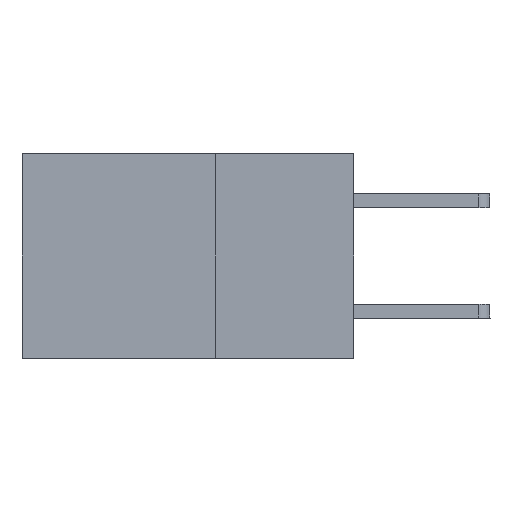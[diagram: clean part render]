
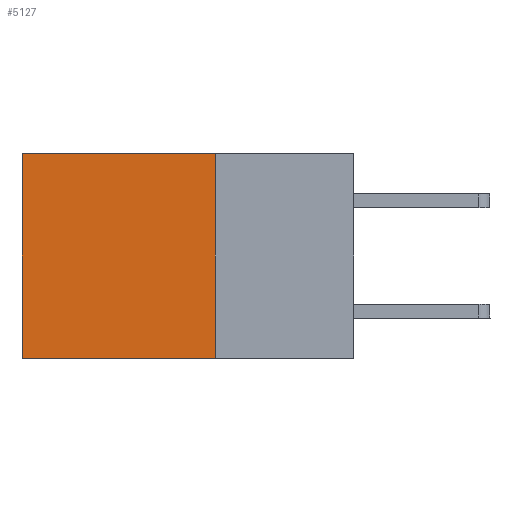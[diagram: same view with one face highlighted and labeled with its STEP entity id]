
A CAD part, left-side view. The second image highlights one B-rep face of the part: STEP entity #5127.
In plain terms, the highlighted planar face has unit normal (-1, 0, 0).
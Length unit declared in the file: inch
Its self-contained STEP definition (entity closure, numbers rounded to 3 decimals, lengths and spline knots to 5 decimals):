
#213 = FACE_OUTER_BOUND ( 'NONE', #970, .T. ) ;
#643 = ORIENTED_EDGE ( 'NONE', *, *, #2461, .T. ) ;
#759 = CARTESIAN_POINT ( 'NONE',  ( 0.2875, 0.25, 0. ) ) ;
#970 = EDGE_LOOP ( 'NONE', ( #4920, #7494, #11373, #643 ) ) ;
#1147 = LINE ( 'NONE', #759, #7965 ) ;
#2006 = CARTESIAN_POINT ( 'NONE',  ( 0.2875, 0.6, -0.37 ) ) ;
#2083 = VECTOR ( 'NONE', #11376, 39.37008 ) ;
#2439 = VERTEX_POINT ( 'NONE', #11408 ) ;
#2461 = EDGE_CURVE ( 'NONE', #11363, #2439, #7066, .T. ) ;
#2597 = CARTESIAN_POINT ( 'NONE',  ( 0.2875, 0.25, -0.37 ) ) ;
#3506 = DIRECTION ( 'NONE',  ( 0., 1., 0. ) ) ;
#4059 = DIRECTION ( 'NONE',  ( 0., 0., -1. ) ) ;
#4685 = VERTEX_POINT ( 'NONE', #2006 ) ;
#4920 = ORIENTED_EDGE ( 'NONE', *, *, #10738, .T. ) ;
#5127 = ADVANCED_FACE ( 'NONE', ( #213 ), #10939, .F. ) ;
#5248 = LINE ( 'NONE', #2597, #7282 ) ;
#5414 = LINE ( 'NONE', #8422, #9764 ) ;
#7003 = VERTEX_POINT ( 'NONE', #9235 ) ;
#7066 = LINE ( 'NONE', #11324, #2083 ) ;
#7282 = VECTOR ( 'NONE', #3506, 39.37008 ) ;
#7494 = ORIENTED_EDGE ( 'NONE', *, *, #10964, .F. ) ;
#7965 = VECTOR ( 'NONE', #10485, 39.37008 ) ;
#8422 = CARTESIAN_POINT ( 'NONE',  ( 0.2875, 0.6, 0. ) ) ;
#8440 = CARTESIAN_POINT ( 'NONE',  ( 0.2875, 0.25, 0. ) ) ;
#9235 = CARTESIAN_POINT ( 'NONE',  ( 0.2875, 0.25, -0.37 ) ) ;
#9301 = DIRECTION ( 'NONE',  ( 1., 0., 0. ) ) ;
#9764 = VECTOR ( 'NONE', #10957, 39.37008 ) ;
#9901 = CARTESIAN_POINT ( 'NONE',  ( 0.2875, 0.25, 0. ) ) ;
#10485 = DIRECTION ( 'NONE',  ( 0., 0., -1. ) ) ;
#10709 = AXIS2_PLACEMENT_3D ( 'NONE', #8440, #9301, #4059 ) ;
#10738 = EDGE_CURVE ( 'NONE', #2439, #4685, #5414, .T. ) ;
#10939 = PLANE ( 'NONE',  #10709 ) ;
#10957 = DIRECTION ( 'NONE',  ( 0., 0., -1. ) ) ;
#10964 = EDGE_CURVE ( 'NONE', #7003, #4685, #5248, .T. ) ;
#11167 = EDGE_CURVE ( 'NONE', #11363, #7003, #1147, .T. ) ;
#11324 = CARTESIAN_POINT ( 'NONE',  ( 0.2875, 0.25, 0. ) ) ;
#11363 = VERTEX_POINT ( 'NONE', #9901 ) ;
#11373 = ORIENTED_EDGE ( 'NONE', *, *, #11167, .F. ) ;
#11376 = DIRECTION ( 'NONE',  ( 0., 1., 0. ) ) ;
#11408 = CARTESIAN_POINT ( 'NONE',  ( 0.2875, 0.6, 0. ) ) ;
